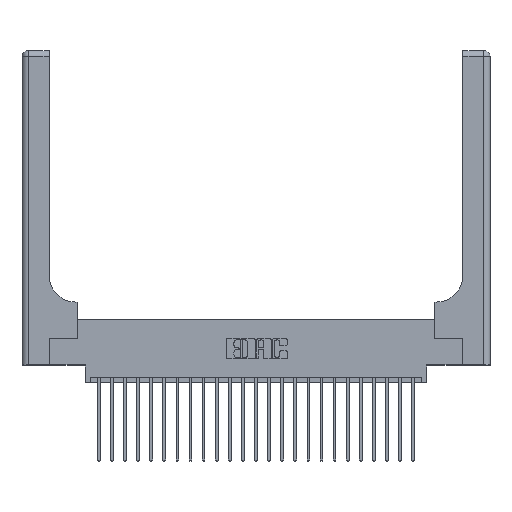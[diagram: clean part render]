
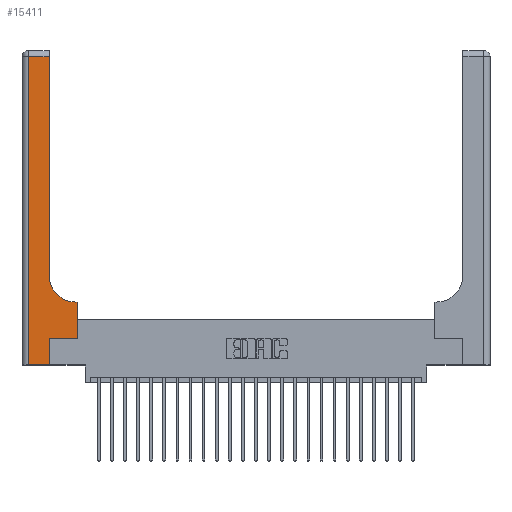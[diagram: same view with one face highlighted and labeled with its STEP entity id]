
A CAD part, top view. The second image highlights one B-rep face of the part: STEP entity #15411.
In plain terms, the highlighted planar face has unit normal (0, 0, 1).
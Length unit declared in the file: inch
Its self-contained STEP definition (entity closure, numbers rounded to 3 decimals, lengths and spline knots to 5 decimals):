
#534 = CARTESIAN_POINT ( 'NONE',  ( 0.265, 0., 0.37 ) ) ;
#555 = ORIENTED_EDGE ( 'NONE', *, *, #14291, .T. ) ;
#776 = DIRECTION ( 'NONE',  ( 1., 0., 0. ) ) ;
#1637 = ORIENTED_EDGE ( 'NONE', *, *, #11437, .T. ) ;
#2405 = DIRECTION ( 'NONE',  ( 0., 1., 0. ) ) ;
#2624 = VERTEX_POINT ( 'NONE', #21970 ) ;
#2945 = FACE_OUTER_BOUND ( 'NONE', #13371, .T. ) ;
#3235 = VECTOR ( 'NONE', #2405, 39.37008 ) ;
#3702 = CARTESIAN_POINT ( 'NONE',  ( 0., 3., 0.37 ) ) ;
#4495 = VERTEX_POINT ( 'NONE', #5997 ) ;
#5546 = CARTESIAN_POINT ( 'NONE',  ( 0.265, 0.25, 0.37 ) ) ;
#5554 = EDGE_CURVE ( 'NONE', #4495, #2624, #11021, .T. ) ;
#5644 = CARTESIAN_POINT ( 'NONE',  ( 0.265, 0., 0.37 ) ) ;
#5997 = CARTESIAN_POINT ( 'NONE',  ( 0.51, 0.6, 0.37 ) ) ;
#6139 = AXIS2_PLACEMENT_3D ( 'NONE', #22010, #10972, #23871 ) ;
#6306 = VERTEX_POINT ( 'NONE', #18098 ) ;
#6409 = VERTEX_POINT ( 'NONE', #18417 ) ;
#6661 = DIRECTION ( 'NONE',  ( -1., 0., 0. ) ) ;
#6668 = VECTOR ( 'NONE', #6661, 39.37008 ) ;
#6869 = DIRECTION ( 'NONE',  ( 0., -1., 0. ) ) ;
#7190 = VERTEX_POINT ( 'NONE', #19267 ) ;
#8197 = LINE ( 'NONE', #8998, #22325 ) ;
#8683 = CARTESIAN_POINT ( 'NONE',  ( 0.06, 2.94, 0.37 ) ) ;
#8876 = LINE ( 'NONE', #18030, #13197 ) ;
#8998 = CARTESIAN_POINT ( 'NONE',  ( 0.265, 0.25, 0.37 ) ) ;
#9407 = DIRECTION ( 'NONE',  ( 0., 0., -1. ) ) ;
#10478 = VECTOR ( 'NONE', #12605, 39.37008 ) ;
#10550 = ORIENTED_EDGE ( 'NONE', *, *, #21153, .T. ) ;
#10879 = VERTEX_POINT ( 'NONE', #17794 ) ;
#10972 = DIRECTION ( 'NONE',  ( 0., 0., -1. ) ) ;
#11021 = CIRCLE ( 'NONE', #6139, 0.25 ) ;
#11219 = LINE ( 'NONE', #17928, #11820 ) ;
#11437 = EDGE_CURVE ( 'NONE', #2624, #6306, #11219, .T. ) ;
#11820 = VECTOR ( 'NONE', #23401, 39.37008 ) ;
#12383 = EDGE_CURVE ( 'NONE', #15157, #7190, #8876, .T. ) ;
#12605 = DIRECTION ( 'NONE',  ( -1., 0., 0. ) ) ;
#12709 = DIRECTION ( 'NONE',  ( 1., 0., 0. ) ) ;
#13197 = VECTOR ( 'NONE', #6869, 39.37008 ) ;
#13359 = VECTOR ( 'NONE', #19546, 39.37008 ) ;
#13371 = EDGE_LOOP ( 'NONE', ( #1637, #10550, #19275, #19097, #21092, #555, #22563, #23529, #19724 ) ) ;
#14021 = CARTESIAN_POINT ( 'NONE',  ( 0.26, 0.6, 0.37 ) ) ;
#14291 = EDGE_CURVE ( 'NONE', #22889, #6409, #8197, .T. ) ;
#15157 = VERTEX_POINT ( 'NONE', #8683 ) ;
#15369 = LINE ( 'NONE', #18081, #10478 ) ;
#15411 = ADVANCED_FACE ( 'NONE', ( #2945 ), #20420, .F. ) ;
#15576 = EDGE_CURVE ( 'NONE', #22536, #22889, #17989, .T. ) ;
#15760 = EDGE_CURVE ( 'NONE', #6409, #10879, #23740, .T. ) ;
#17794 = CARTESIAN_POINT ( 'NONE',  ( 0.528, 0.6, 0.37 ) ) ;
#17928 = CARTESIAN_POINT ( 'NONE',  ( 0.26, 3., 0.37 ) ) ;
#17989 = LINE ( 'NONE', #534, #3235 ) ;
#18030 = CARTESIAN_POINT ( 'NONE',  ( 0.06, 3., 0.37 ) ) ;
#18081 = CARTESIAN_POINT ( 'NONE',  ( 0., 2.94, 0.37 ) ) ;
#18098 = CARTESIAN_POINT ( 'NONE',  ( 0.26, 2.94, 0.37 ) ) ;
#18417 = CARTESIAN_POINT ( 'NONE',  ( 0.528, 0.25, 0.37 ) ) ;
#18742 = AXIS2_PLACEMENT_3D ( 'NONE', #3702, #9407, #22291 ) ;
#18842 = VECTOR ( 'NONE', #776, 39.37008 ) ;
#19097 = ORIENTED_EDGE ( 'NONE', *, *, #21003, .T. ) ;
#19267 = CARTESIAN_POINT ( 'NONE',  ( 0.06, 0., 0.37 ) ) ;
#19275 = ORIENTED_EDGE ( 'NONE', *, *, #12383, .T. ) ;
#19456 = CARTESIAN_POINT ( 'NONE',  ( 0.528, 0.25, 0.37 ) ) ;
#19546 = DIRECTION ( 'NONE',  ( 0., 1., 0. ) ) ;
#19724 = ORIENTED_EDGE ( 'NONE', *, *, #5554, .T. ) ;
#20420 = PLANE ( 'NONE',  #18742 ) ;
#20817 = LINE ( 'NONE', #14021, #6668 ) ;
#21003 = EDGE_CURVE ( 'NONE', #7190, #22536, #23741, .T. ) ;
#21092 = ORIENTED_EDGE ( 'NONE', *, *, #15576, .T. ) ;
#21153 = EDGE_CURVE ( 'NONE', #6306, #15157, #15369, .T. ) ;
#21635 = EDGE_CURVE ( 'NONE', #10879, #4495, #20817, .T. ) ;
#21970 = CARTESIAN_POINT ( 'NONE',  ( 0.26, 0.85, 0.37 ) ) ;
#22010 = CARTESIAN_POINT ( 'NONE',  ( 0.51, 0.85, 0.37 ) ) ;
#22291 = DIRECTION ( 'NONE',  ( -1., 0., 0. ) ) ;
#22325 = VECTOR ( 'NONE', #12709, 39.37008 ) ;
#22536 = VERTEX_POINT ( 'NONE', #5644 ) ;
#22563 = ORIENTED_EDGE ( 'NONE', *, *, #15760, .T. ) ;
#22889 = VERTEX_POINT ( 'NONE', #5546 ) ;
#22922 = CARTESIAN_POINT ( 'NONE',  ( 0., 0., 0.37 ) ) ;
#23401 = DIRECTION ( 'NONE',  ( 0., 1., 0. ) ) ;
#23529 = ORIENTED_EDGE ( 'NONE', *, *, #21635, .T. ) ;
#23740 = LINE ( 'NONE', #19456, #13359 ) ;
#23741 = LINE ( 'NONE', #22922, #18842 ) ;
#23871 = DIRECTION ( 'NONE',  ( 1., 0., 0. ) ) ;
